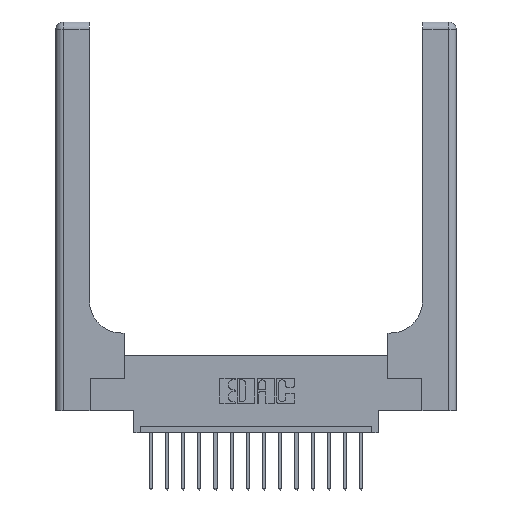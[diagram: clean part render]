
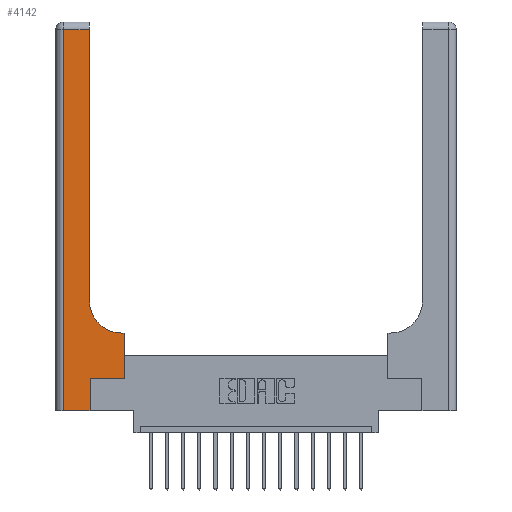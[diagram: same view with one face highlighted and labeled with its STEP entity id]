
A CAD part, top view. The second image highlights one B-rep face of the part: STEP entity #4142.
In plain terms, the highlighted planar face has unit normal (0, 0, 1).
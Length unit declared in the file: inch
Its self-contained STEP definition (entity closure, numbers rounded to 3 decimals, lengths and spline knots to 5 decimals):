
#921 = EDGE_CURVE ( 'NONE', #10398, #16373, #13523, .T. ) ;
#1060 = EDGE_CURVE ( 'NONE', #9895, #10398, #17194, .T. ) ;
#1069 = CARTESIAN_POINT ( 'NONE',  ( 0., 2.94, 0.37 ) ) ;
#1230 = VERTEX_POINT ( 'NONE', #6420 ) ;
#1237 = DIRECTION ( 'NONE',  ( 0., 0., -1. ) ) ;
#1405 = LINE ( 'NONE', #12810, #11735 ) ;
#1494 = DIRECTION ( 'NONE',  ( 0., 1., 0. ) ) ;
#1872 = VERTEX_POINT ( 'NONE', #5974 ) ;
#3037 = VERTEX_POINT ( 'NONE', #14026 ) ;
#3344 = ORIENTED_EDGE ( 'NONE', *, *, #14777, .T. ) ;
#3347 = VECTOR ( 'NONE', #6717, 39.37008 ) ;
#3441 = CARTESIAN_POINT ( 'NONE',  ( 0.265, 0.25, 0.37 ) ) ;
#3450 = AXIS2_PLACEMENT_3D ( 'NONE', #13844, #1237, #16458 ) ;
#3568 = CARTESIAN_POINT ( 'NONE',  ( 0.265, 0.25, 0.37 ) ) ;
#3697 = VECTOR ( 'NONE', #6888, 39.37008 ) ;
#3731 = ORIENTED_EDGE ( 'NONE', *, *, #15678, .T. ) ;
#4074 = EDGE_CURVE ( 'NONE', #3037, #1230, #15512, .T. ) ;
#4142 = ADVANCED_FACE ( 'NONE', ( #11637 ), #8776, .F. ) ;
#4174 = VERTEX_POINT ( 'NONE', #15884 ) ;
#4304 = LINE ( 'NONE', #14162, #3697 ) ;
#4367 = DIRECTION ( 'NONE',  ( -1., 0., 0. ) ) ;
#4630 = EDGE_CURVE ( 'NONE', #16373, #4174, #1405, .T. ) ;
#4768 = ORIENTED_EDGE ( 'NONE', *, *, #1060, .T. ) ;
#5974 = CARTESIAN_POINT ( 'NONE',  ( 0.26, 2.94, 0.37 ) ) ;
#6001 = CARTESIAN_POINT ( 'NONE',  ( 0.26, 3., 0.37 ) ) ;
#6160 = VERTEX_POINT ( 'NONE', #13288 ) ;
#6402 = CARTESIAN_POINT ( 'NONE',  ( 0.528, 0.25, 0.37 ) ) ;
#6420 = CARTESIAN_POINT ( 'NONE',  ( 0.26, 0.85, 0.37 ) ) ;
#6504 = DIRECTION ( 'NONE',  ( -1., 0., 0. ) ) ;
#6717 = DIRECTION ( 'NONE',  ( 1., 0., 0. ) ) ;
#6888 = DIRECTION ( 'NONE',  ( 1., 0., 0. ) ) ;
#8156 = CARTESIAN_POINT ( 'NONE',  ( 0.265, 0., 0.37 ) ) ;
#8384 = VECTOR ( 'NONE', #11362, 39.37008 ) ;
#8776 = PLANE ( 'NONE',  #16119 ) ;
#9726 = LINE ( 'NONE', #1069, #13666 ) ;
#9895 = VERTEX_POINT ( 'NONE', #8156 ) ;
#10296 = VECTOR ( 'NONE', #6504, 39.37008 ) ;
#10377 = ORIENTED_EDGE ( 'NONE', *, *, #921, .T. ) ;
#10398 = VERTEX_POINT ( 'NONE', #3441 ) ;
#10404 = VECTOR ( 'NONE', #12397, 39.37008 ) ;
#10654 = CARTESIAN_POINT ( 'NONE',  ( 0.26, 0.6, 0.37 ) ) ;
#11319 = VECTOR ( 'NONE', #17293, 39.37008 ) ;
#11362 = DIRECTION ( 'NONE',  ( 0., 1., 0. ) ) ;
#11637 = FACE_OUTER_BOUND ( 'NONE', #13099, .T. ) ;
#11646 = EDGE_CURVE ( 'NONE', #4174, #3037, #17828, .T. ) ;
#11735 = VECTOR ( 'NONE', #1494, 39.37008 ) ;
#12397 = DIRECTION ( 'NONE',  ( 0., -1., 0. ) ) ;
#12475 = CARTESIAN_POINT ( 'NONE',  ( 0.06, 3., 0.37 ) ) ;
#12569 = LINE ( 'NONE', #12475, #10404 ) ;
#12810 = CARTESIAN_POINT ( 'NONE',  ( 0.528, 0.25, 0.37 ) ) ;
#12848 = EDGE_CURVE ( 'NONE', #6160, #17213, #12569, .T. ) ;
#12864 = CARTESIAN_POINT ( 'NONE',  ( 0.265, 0., 0.37 ) ) ;
#13099 = EDGE_LOOP ( 'NONE', ( #16045, #3344, #16335, #3731, #4768, #10377, #15364, #15857, #14532 ) ) ;
#13288 = CARTESIAN_POINT ( 'NONE',  ( 0.06, 2.94, 0.37 ) ) ;
#13343 = CARTESIAN_POINT ( 'NONE',  ( 0.06, 0., 0.37 ) ) ;
#13523 = LINE ( 'NONE', #3568, #3347 ) ;
#13666 = VECTOR ( 'NONE', #16639, 39.37008 ) ;
#13844 = CARTESIAN_POINT ( 'NONE',  ( 0.51, 0.85, 0.37 ) ) ;
#14026 = CARTESIAN_POINT ( 'NONE',  ( 0.51, 0.6, 0.37 ) ) ;
#14031 = DIRECTION ( 'NONE',  ( 0., 0., -1. ) ) ;
#14162 = CARTESIAN_POINT ( 'NONE',  ( 0., 0., 0.37 ) ) ;
#14388 = LINE ( 'NONE', #6001, #8384 ) ;
#14532 = ORIENTED_EDGE ( 'NONE', *, *, #4074, .T. ) ;
#14777 = EDGE_CURVE ( 'NONE', #1872, #6160, #9726, .T. ) ;
#15324 = EDGE_CURVE ( 'NONE', #1230, #1872, #14388, .T. ) ;
#15364 = ORIENTED_EDGE ( 'NONE', *, *, #4630, .T. ) ;
#15512 = CIRCLE ( 'NONE', #3450, 0.25 ) ;
#15678 = EDGE_CURVE ( 'NONE', #17213, #9895, #4304, .T. ) ;
#15796 = CARTESIAN_POINT ( 'NONE',  ( 0., 3., 0.37 ) ) ;
#15857 = ORIENTED_EDGE ( 'NONE', *, *, #11646, .T. ) ;
#15884 = CARTESIAN_POINT ( 'NONE',  ( 0.528, 0.6, 0.37 ) ) ;
#16045 = ORIENTED_EDGE ( 'NONE', *, *, #15324, .T. ) ;
#16119 = AXIS2_PLACEMENT_3D ( 'NONE', #15796, #14031, #4367 ) ;
#16335 = ORIENTED_EDGE ( 'NONE', *, *, #12848, .T. ) ;
#16373 = VERTEX_POINT ( 'NONE', #6402 ) ;
#16458 = DIRECTION ( 'NONE',  ( 1., 0., 0. ) ) ;
#16639 = DIRECTION ( 'NONE',  ( -1., 0., 0. ) ) ;
#17194 = LINE ( 'NONE', #12864, #11319 ) ;
#17213 = VERTEX_POINT ( 'NONE', #13343 ) ;
#17293 = DIRECTION ( 'NONE',  ( 0., 1., 0. ) ) ;
#17828 = LINE ( 'NONE', #10654, #10296 ) ;
